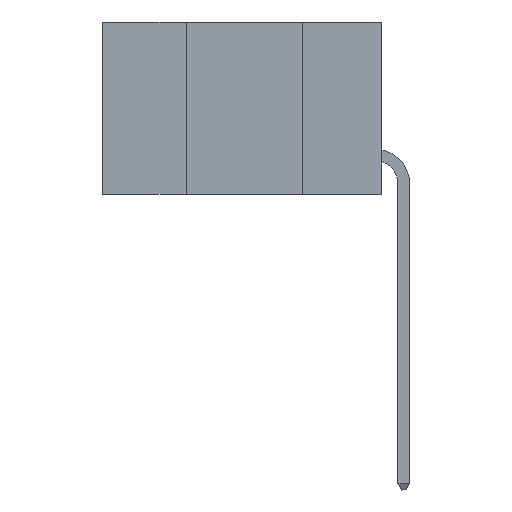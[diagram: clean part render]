
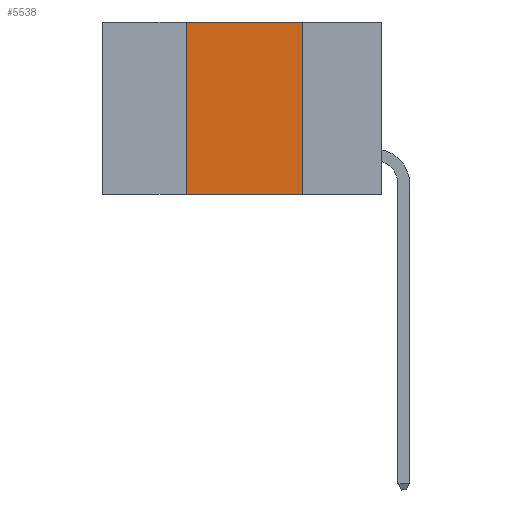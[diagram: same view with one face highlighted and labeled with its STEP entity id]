
A CAD part, left-side view. The second image highlights one B-rep face of the part: STEP entity #5538.
In plain terms, the highlighted planar face has unit normal (-1, 0, 0).
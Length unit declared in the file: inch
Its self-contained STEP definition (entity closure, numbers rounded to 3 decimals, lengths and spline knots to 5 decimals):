
#415 = ORIENTED_EDGE ( 'NONE', *, *, #6741, .F. ) ;
#1166 = EDGE_CURVE ( 'NONE', #5205, #11725, #2054, .T. ) ;
#1279 = PLANE ( 'NONE',  #3939 ) ;
#1356 = CARTESIAN_POINT ( 'NONE',  ( 0., 0.17, 0. ) ) ;
#1405 = VERTEX_POINT ( 'NONE', #4097 ) ;
#2054 = LINE ( 'NONE', #5889, #9950 ) ;
#3181 = VECTOR ( 'NONE', #11769, 39.37008 ) ;
#3544 = DIRECTION ( 'NONE',  ( 0., 0., -1. ) ) ;
#3591 = ORIENTED_EDGE ( 'NONE', *, *, #1166, .T. ) ;
#3723 = VERTEX_POINT ( 'NONE', #3969 ) ;
#3939 = AXIS2_PLACEMENT_3D ( 'NONE', #8045, #9107, #3544 ) ;
#3969 = CARTESIAN_POINT ( 'NONE',  ( 0., 0.17, 0. ) ) ;
#4097 = CARTESIAN_POINT ( 'NONE',  ( 0., 0.42, 0. ) ) ;
#5205 = VERTEX_POINT ( 'NONE', #11544 ) ;
#5538 = ADVANCED_FACE ( 'NONE', ( #13472 ), #1279, .F. ) ;
#5889 = CARTESIAN_POINT ( 'NONE',  ( 0., 0.6, -0.37 ) ) ;
#5943 = EDGE_LOOP ( 'NONE', ( #415, #9616, #9376, #3591 ) ) ;
#6026 = CARTESIAN_POINT ( 'NONE',  ( 0., 0.17, -0.37 ) ) ;
#6145 = CARTESIAN_POINT ( 'NONE',  ( 0., 0.6, 0. ) ) ;
#6741 = EDGE_CURVE ( 'NONE', #3723, #11725, #9968, .T. ) ;
#7381 = VECTOR ( 'NONE', #11885, 39.37008 ) ;
#7495 = VECTOR ( 'NONE', #11443, 39.37008 ) ;
#8045 = CARTESIAN_POINT ( 'NONE',  ( 0., 0.6, 0. ) ) ;
#9107 = DIRECTION ( 'NONE',  ( 1., 0., 0. ) ) ;
#9268 = DIRECTION ( 'NONE',  ( 0., -1., 0. ) ) ;
#9376 = ORIENTED_EDGE ( 'NONE', *, *, #12867, .F. ) ;
#9616 = ORIENTED_EDGE ( 'NONE', *, *, #13608, .F. ) ;
#9950 = VECTOR ( 'NONE', #9268, 39.37008 ) ;
#9968 = LINE ( 'NONE', #1356, #7495 ) ;
#10892 = LINE ( 'NONE', #12872, #7381 ) ;
#11443 = DIRECTION ( 'NONE',  ( 0., 0., -1. ) ) ;
#11544 = CARTESIAN_POINT ( 'NONE',  ( 0., 0.42, -0.37 ) ) ;
#11725 = VERTEX_POINT ( 'NONE', #6026 ) ;
#11769 = DIRECTION ( 'NONE',  ( 0., -1., 0. ) ) ;
#11885 = DIRECTION ( 'NONE',  ( 0., 0., 1. ) ) ;
#12867 = EDGE_CURVE ( 'NONE', #5205, #1405, #10892, .T. ) ;
#12872 = CARTESIAN_POINT ( 'NONE',  ( 0., 0.42, 0. ) ) ;
#13152 = LINE ( 'NONE', #6145, #3181 ) ;
#13472 = FACE_OUTER_BOUND ( 'NONE', #5943, .T. ) ;
#13608 = EDGE_CURVE ( 'NONE', #1405, #3723, #13152, .T. ) ;
